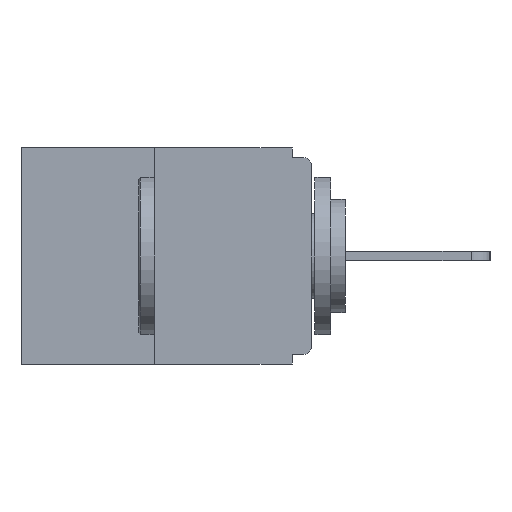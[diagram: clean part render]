
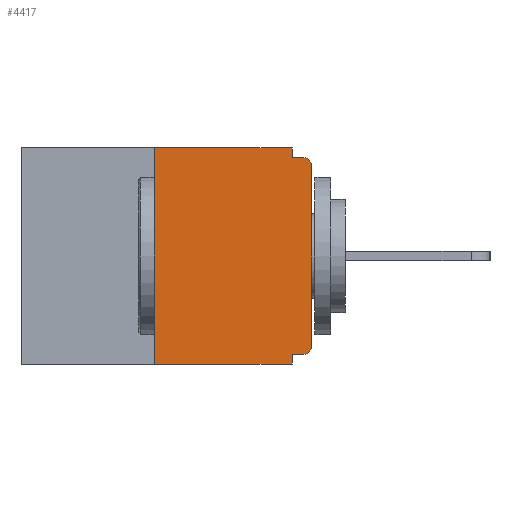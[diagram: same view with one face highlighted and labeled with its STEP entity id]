
A CAD part, left-side view. The second image highlights one B-rep face of the part: STEP entity #4417.
In plain terms, the highlighted planar face has unit normal (-1, 0, 0).
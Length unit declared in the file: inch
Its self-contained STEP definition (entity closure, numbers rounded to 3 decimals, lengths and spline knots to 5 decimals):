
#20 = CARTESIAN_POINT ( 'NONE',  ( 0., 0.015, -0.015 ) ) ;
#314 = ORIENTED_EDGE ( 'NONE', *, *, #17816, .F. ) ;
#616 = ORIENTED_EDGE ( 'NONE', *, *, #12624, .T. ) ;
#844 = VECTOR ( 'NONE', #20635, 39.37008 ) ;
#1077 = ORIENTED_EDGE ( 'NONE', *, *, #4216, .F. ) ;
#1084 = LINE ( 'NONE', #26456, #13081 ) ;
#1130 = EDGE_LOOP ( 'NONE', ( #12090, #18944, #8575, #314, #1077, #19593, #616, #7061, #17847, #21982 ) ) ;
#1686 = CARTESIAN_POINT ( 'NONE',  ( 0., 0., -0.03 ) ) ;
#2440 = DIRECTION ( 'NONE',  ( 1., 0., 0. ) ) ;
#2536 = VERTEX_POINT ( 'NONE', #25721 ) ;
#2724 = EDGE_CURVE ( 'NONE', #10362, #12379, #13986, .T. ) ;
#4216 = EDGE_CURVE ( 'NONE', #2536, #18280, #1084, .T. ) ;
#4417 = ADVANCED_FACE ( 'NONE', ( #13319 ), #23647, .F. ) ;
#4425 = LINE ( 'NONE', #19055, #14792 ) ;
#5030 = VERTEX_POINT ( 'NONE', #25538 ) ;
#6504 = CARTESIAN_POINT ( 'NONE',  ( 0., 0.031, -0.015 ) ) ;
#6767 = VECTOR ( 'NONE', #10381, 39.37008 ) ;
#7061 = ORIENTED_EDGE ( 'NONE', *, *, #11581, .T. ) ;
#7451 = VECTOR ( 'NONE', #9537, 39.37008 ) ;
#7494 = DIRECTION ( 'NONE',  ( 0., 1., 0. ) ) ;
#7794 = EDGE_CURVE ( 'NONE', #5030, #23972, #4425, .T. ) ;
#8215 = CARTESIAN_POINT ( 'NONE',  ( 0., 0., -0.313 ) ) ;
#8345 = CARTESIAN_POINT ( 'NONE',  ( 0., 0.25, 0. ) ) ;
#8409 = CARTESIAN_POINT ( 'NONE',  ( 0., 0., -0.015 ) ) ;
#8575 = ORIENTED_EDGE ( 'NONE', *, *, #14359, .T. ) ;
#8600 = DIRECTION ( 'NONE',  ( 0., 0., -1. ) ) ;
#9215 = AXIS2_PLACEMENT_3D ( 'NONE', #19664, #15482, #12982 ) ;
#9455 = DIRECTION ( 'NONE',  ( 0., 0., -1. ) ) ;
#9537 = DIRECTION ( 'NONE',  ( 0., -1., 0. ) ) ;
#10232 = CARTESIAN_POINT ( 'NONE',  ( 0., 0.031, 0. ) ) ;
#10362 = VERTEX_POINT ( 'NONE', #6504 ) ;
#10381 = DIRECTION ( 'NONE',  ( 0., -1., 0. ) ) ;
#10672 = VECTOR ( 'NONE', #21008, 39.37008 ) ;
#11105 = CARTESIAN_POINT ( 'NONE',  ( 0., 0.46, 0. ) ) ;
#11308 = CIRCLE ( 'NONE', #15743, 0.015 ) ;
#11581 = EDGE_CURVE ( 'NONE', #23475, #12379, #11308, .T. ) ;
#11623 = LINE ( 'NONE', #20110, #7451 ) ;
#11707 = LINE ( 'NONE', #26624, #21228 ) ;
#12090 = ORIENTED_EDGE ( 'NONE', *, *, #16086, .F. ) ;
#12204 = AXIS2_PLACEMENT_3D ( 'NONE', #11105, #2440, #21686 ) ;
#12236 = CARTESIAN_POINT ( 'NONE',  ( 0., 0., 0. ) ) ;
#12379 = VERTEX_POINT ( 'NONE', #20 ) ;
#12624 = EDGE_CURVE ( 'NONE', #19253, #23475, #25202, .T. ) ;
#12923 = DIRECTION ( 'NONE',  ( 0., 0., 1. ) ) ;
#12982 = DIRECTION ( 'NONE',  ( 0., 0., -1. ) ) ;
#13081 = VECTOR ( 'NONE', #7494, 39.37008 ) ;
#13319 = FACE_OUTER_BOUND ( 'NONE', #1130, .T. ) ;
#13986 = LINE ( 'NONE', #8409, #6767 ) ;
#14359 = EDGE_CURVE ( 'NONE', #5030, #17861, #11707, .T. ) ;
#14792 = VECTOR ( 'NONE', #12923, 39.37008 ) ;
#15290 = CARTESIAN_POINT ( 'NONE',  ( 0., 0.015, -0.03 ) ) ;
#15482 = DIRECTION ( 'NONE',  ( -1., 0., 0. ) ) ;
#15743 = AXIS2_PLACEMENT_3D ( 'NONE', #15290, #17923, #9455 ) ;
#16086 = EDGE_CURVE ( 'NONE', #23972, #16113, #11623, .T. ) ;
#16113 = VERTEX_POINT ( 'NONE', #10232 ) ;
#17816 = EDGE_CURVE ( 'NONE', #18280, #17861, #18934, .T. ) ;
#17847 = ORIENTED_EDGE ( 'NONE', *, *, #2724, .F. ) ;
#17861 = VERTEX_POINT ( 'NONE', #25115 ) ;
#17923 = DIRECTION ( 'NONE',  ( -1., 0., 0. ) ) ;
#18280 = VERTEX_POINT ( 'NONE', #22718 ) ;
#18934 = LINE ( 'NONE', #23154, #844 ) ;
#18944 = ORIENTED_EDGE ( 'NONE', *, *, #7794, .F. ) ;
#19055 = CARTESIAN_POINT ( 'NONE',  ( 0., 0.25, 0. ) ) ;
#19253 = VERTEX_POINT ( 'NONE', #8215 ) ;
#19593 = ORIENTED_EDGE ( 'NONE', *, *, #22125, .T. ) ;
#19664 = CARTESIAN_POINT ( 'NONE',  ( 0., 0.015, -0.313 ) ) ;
#20110 = CARTESIAN_POINT ( 'NONE',  ( 0., 0.46, 0. ) ) ;
#20635 = DIRECTION ( 'NONE',  ( 0., 0., -1. ) ) ;
#20868 = CARTESIAN_POINT ( 'NONE',  ( 0., 0.031, 0. ) ) ;
#21008 = DIRECTION ( 'NONE',  ( 0., 0., 1. ) ) ;
#21225 = CIRCLE ( 'NONE', #9215, 0.015 ) ;
#21228 = VECTOR ( 'NONE', #26477, 39.37008 ) ;
#21686 = DIRECTION ( 'NONE',  ( 0., 0., -1. ) ) ;
#21982 = ORIENTED_EDGE ( 'NONE', *, *, #27268, .F. ) ;
#22125 = EDGE_CURVE ( 'NONE', #2536, #19253, #21225, .T. ) ;
#22718 = CARTESIAN_POINT ( 'NONE',  ( 0., 0.031, -0.328 ) ) ;
#22758 = VECTOR ( 'NONE', #8600, 39.37008 ) ;
#22848 = LINE ( 'NONE', #20868, #22758 ) ;
#23154 = CARTESIAN_POINT ( 'NONE',  ( 0., 0.031, -0.343 ) ) ;
#23475 = VERTEX_POINT ( 'NONE', #1686 ) ;
#23647 = PLANE ( 'NONE',  #12204 ) ;
#23972 = VERTEX_POINT ( 'NONE', #8345 ) ;
#25115 = CARTESIAN_POINT ( 'NONE',  ( 0., 0.031, -0.343 ) ) ;
#25202 = LINE ( 'NONE', #12236, #10672 ) ;
#25538 = CARTESIAN_POINT ( 'NONE',  ( 0., 0.25, -0.343 ) ) ;
#25721 = CARTESIAN_POINT ( 'NONE',  ( 0., 0.015, -0.328 ) ) ;
#26456 = CARTESIAN_POINT ( 'NONE',  ( 0., 0., -0.328 ) ) ;
#26477 = DIRECTION ( 'NONE',  ( 0., -1., 0. ) ) ;
#26624 = CARTESIAN_POINT ( 'NONE',  ( 0., 0.46, -0.343 ) ) ;
#27268 = EDGE_CURVE ( 'NONE', #16113, #10362, #22848, .T. ) ;
